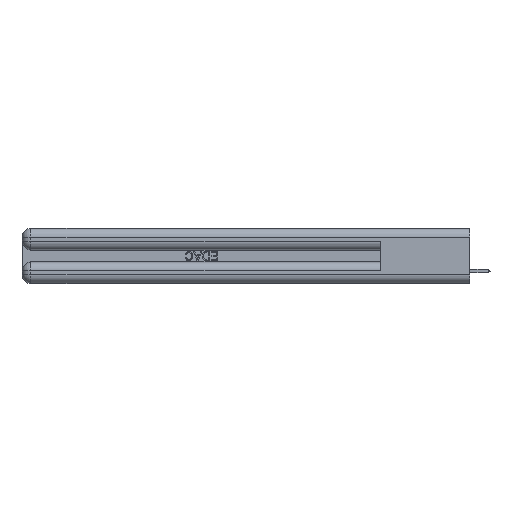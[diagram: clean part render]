
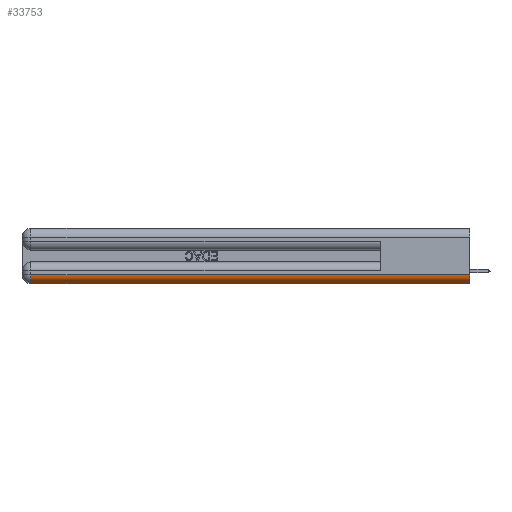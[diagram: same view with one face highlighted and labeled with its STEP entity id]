
A CAD part, left-side view. The second image highlights one B-rep face of the part: STEP entity #33753.
In plain terms, the highlighted cylindrical face has radius 1.524 mm (diameter 3.048 mm), a partial arc.
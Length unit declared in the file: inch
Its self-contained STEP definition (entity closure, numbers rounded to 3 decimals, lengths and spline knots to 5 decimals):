
#902 = EDGE_CURVE ( 'NONE', #19956, #11134, #8822, .T. ) ;
#3854 = VECTOR ( 'NONE', #40117, 39.37008 ) ;
#3876 = CARTESIAN_POINT ( 'NONE',  ( 0.06, 3., 0. ) ) ;
#4259 = EDGE_CURVE ( 'NONE', #11134, #28091, #30554, .T. ) ;
#5299 = VECTOR ( 'NONE', #39732, 39.37008 ) ;
#6708 = FACE_OUTER_BOUND ( 'NONE', #18992, .T. ) ;
#8822 = LINE ( 'NONE', #34581, #3854 ) ;
#9355 = AXIS2_PLACEMENT_3D ( 'NONE', #10719, #10448, #14024 ) ;
#10448 = DIRECTION ( 'NONE',  ( 0., -1., 0. ) ) ;
#10719 = CARTESIAN_POINT ( 'NONE',  ( 0.06, 0., 0.06 ) ) ;
#11095 = AXIS2_PLACEMENT_3D ( 'NONE', #16996, #20487, #44975 ) ;
#11134 = VERTEX_POINT ( 'NONE', #22294 ) ;
#12454 = ORIENTED_EDGE ( 'NONE', *, *, #902, .F. ) ;
#14024 = DIRECTION ( 'NONE',  ( 0., 0., 1. ) ) ;
#14907 = EDGE_CURVE ( 'NONE', #28091, #27762, #42577, .T. ) ;
#16101 = CARTESIAN_POINT ( 'NONE',  ( 0.06, 2.94, 0. ) ) ;
#16443 = AXIS2_PLACEMENT_3D ( 'NONE', #26482, #44268, #43950 ) ;
#16996 = CARTESIAN_POINT ( 'NONE',  ( 0.06, 0., 0.06 ) ) ;
#17656 = CYLINDRICAL_SURFACE ( 'NONE', #11095, 0.06 ) ;
#18992 = EDGE_LOOP ( 'NONE', ( #31585, #12454, #39382, #25089 ) ) ;
#19423 = CARTESIAN_POINT ( 'NONE',  ( 0.06, 0., 0. ) ) ;
#19956 = VERTEX_POINT ( 'NONE', #25338 ) ;
#20487 = DIRECTION ( 'NONE',  ( 0., 1., 0. ) ) ;
#22294 = CARTESIAN_POINT ( 'NONE',  ( 0., 0., 0.06 ) ) ;
#25089 = ORIENTED_EDGE ( 'NONE', *, *, #14907, .F. ) ;
#25338 = CARTESIAN_POINT ( 'NONE',  ( 0., 2.94, 0.06 ) ) ;
#26482 = CARTESIAN_POINT ( 'NONE',  ( 0.06, 2.94, 0.06 ) ) ;
#27711 = EDGE_CURVE ( 'NONE', #27762, #19956, #34919, .T. ) ;
#27762 = VERTEX_POINT ( 'NONE', #16101 ) ;
#28091 = VERTEX_POINT ( 'NONE', #19423 ) ;
#30554 = CIRCLE ( 'NONE', #9355, 0.06 ) ;
#31585 = ORIENTED_EDGE ( 'NONE', *, *, #4259, .F. ) ;
#33753 = ADVANCED_FACE ( 'NONE', ( #6708 ), #17656, .T. ) ;
#34581 = CARTESIAN_POINT ( 'NONE',  ( 0., 0., 0.06 ) ) ;
#34919 = CIRCLE ( 'NONE', #16443, 0.06 ) ;
#39382 = ORIENTED_EDGE ( 'NONE', *, *, #27711, .F. ) ;
#39732 = DIRECTION ( 'NONE',  ( 0., 1., 0. ) ) ;
#40117 = DIRECTION ( 'NONE',  ( 0., -1., 0. ) ) ;
#42577 = LINE ( 'NONE', #3876, #5299 ) ;
#43950 = DIRECTION ( 'NONE',  ( 0., 0., 1. ) ) ;
#44268 = DIRECTION ( 'NONE',  ( 0., 1., 0. ) ) ;
#44975 = DIRECTION ( 'NONE',  ( 0., 0., 1. ) ) ;
